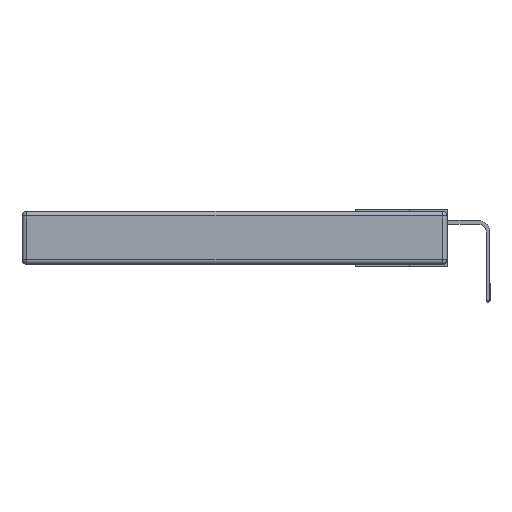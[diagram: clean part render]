
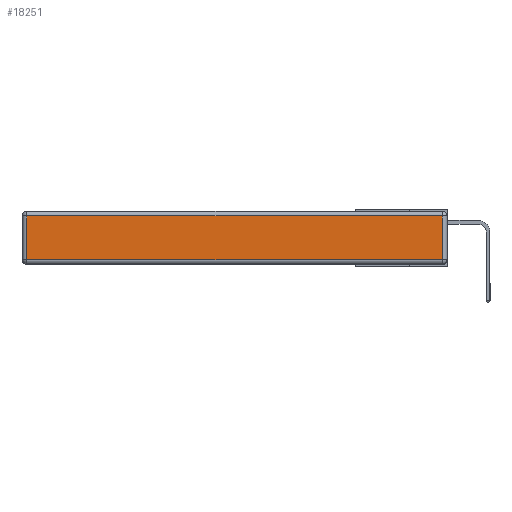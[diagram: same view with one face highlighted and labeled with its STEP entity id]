
A CAD part, left-side view. The second image highlights one B-rep face of the part: STEP entity #18251.
In plain terms, the highlighted planar face has unit normal (-1, 0, 0).
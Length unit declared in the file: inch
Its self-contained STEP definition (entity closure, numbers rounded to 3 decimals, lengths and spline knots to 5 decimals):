
#950 = VERTEX_POINT ( 'NONE', #17541 ) ;
#1303 = EDGE_CURVE ( 'NONE', #14730, #950, #14306, .T. ) ;
#2285 = CARTESIAN_POINT ( 'NONE',  ( 0., 2.72, -0.313 ) ) ;
#2312 = CARTESIAN_POINT ( 'NONE',  ( 0., 2.75, -0.03 ) ) ;
#2456 = DIRECTION ( 'NONE',  ( 0., 0., 1. ) ) ;
#2808 = ORIENTED_EDGE ( 'NONE', *, *, #3994, .T. ) ;
#3386 = CARTESIAN_POINT ( 'NONE',  ( 0., 0., -0.343 ) ) ;
#3994 = EDGE_CURVE ( 'NONE', #17155, #8625, #16473, .T. ) ;
#4294 = CARTESIAN_POINT ( 'NONE',  ( 0., 2.72, -0.03 ) ) ;
#4400 = AXIS2_PLACEMENT_3D ( 'NONE', #3386, #13507, #4855 ) ;
#4855 = DIRECTION ( 'NONE',  ( 0., 0., 1. ) ) ;
#6269 = EDGE_CURVE ( 'NONE', #950, #17155, #9395, .T. ) ;
#6368 = PLANE ( 'NONE',  #4400 ) ;
#6706 = DIRECTION ( 'NONE',  ( 0., -1., 0. ) ) ;
#7982 = VECTOR ( 'NONE', #6706, 39.37008 ) ;
#8143 = CARTESIAN_POINT ( 'NONE',  ( 0., 2.72, -0.343 ) ) ;
#8625 = VERTEX_POINT ( 'NONE', #4294 ) ;
#9395 = LINE ( 'NONE', #18328, #15741 ) ;
#9588 = DIRECTION ( 'NONE',  ( 0., 0., -1. ) ) ;
#11109 = CARTESIAN_POINT ( 'NONE',  ( 0., 0.03, -0.03 ) ) ;
#11683 = LINE ( 'NONE', #8143, #12812 ) ;
#11711 = ORIENTED_EDGE ( 'NONE', *, *, #6269, .T. ) ;
#12397 = DIRECTION ( 'NONE',  ( 0., 1., 0. ) ) ;
#12576 = EDGE_CURVE ( 'NONE', #8625, #14730, #11683, .T. ) ;
#12812 = VECTOR ( 'NONE', #9588, 39.37008 ) ;
#13439 = EDGE_LOOP ( 'NONE', ( #15485, #11711, #2808, #13772 ) ) ;
#13507 = DIRECTION ( 'NONE',  ( -1., 0., 0. ) ) ;
#13772 = ORIENTED_EDGE ( 'NONE', *, *, #12576, .T. ) ;
#13885 = CARTESIAN_POINT ( 'NONE',  ( 0., 0., -0.313 ) ) ;
#14306 = LINE ( 'NONE', #13885, #7982 ) ;
#14730 = VERTEX_POINT ( 'NONE', #2285 ) ;
#15485 = ORIENTED_EDGE ( 'NONE', *, *, #1303, .T. ) ;
#15741 = VECTOR ( 'NONE', #2456, 39.37008 ) ;
#16473 = LINE ( 'NONE', #2312, #16909 ) ;
#16888 = FACE_OUTER_BOUND ( 'NONE', #13439, .T. ) ;
#16909 = VECTOR ( 'NONE', #12397, 39.37008 ) ;
#17155 = VERTEX_POINT ( 'NONE', #11109 ) ;
#17541 = CARTESIAN_POINT ( 'NONE',  ( 0., 0.03, -0.313 ) ) ;
#18251 = ADVANCED_FACE ( 'NONE', ( #16888 ), #6368, .T. ) ;
#18328 = CARTESIAN_POINT ( 'NONE',  ( 0., 0.03, -0.343 ) ) ;
